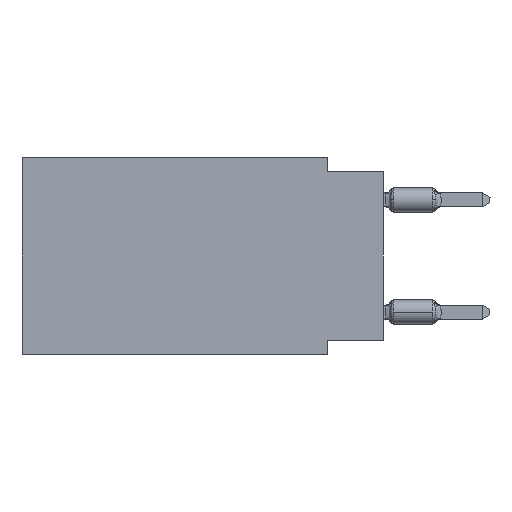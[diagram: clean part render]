
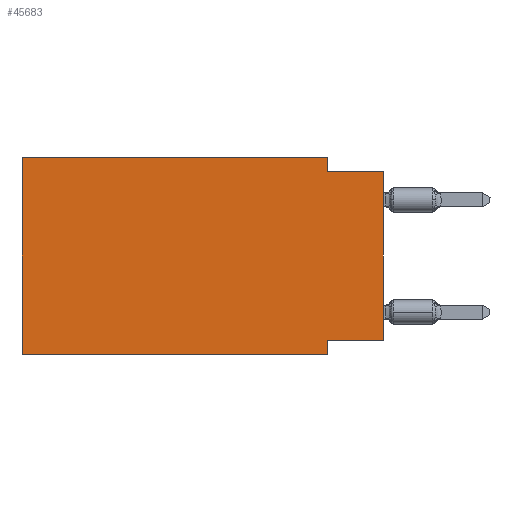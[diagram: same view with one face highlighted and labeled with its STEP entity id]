
A CAD part, left-side view. The second image highlights one B-rep face of the part: STEP entity #45683.
In plain terms, the highlighted planar face has unit normal (-1, 0, 0).
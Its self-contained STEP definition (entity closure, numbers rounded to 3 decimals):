
#59 = DIRECTION ( 'NONE',  ( 0., 0., -1. ) ) ;
#446 = FACE_OUTER_BOUND ( 'NONE', #4276, .T. ) ;
#1036 = LINE ( 'NONE', #35145, #41183 ) ;
#1537 = VECTOR ( 'NONE', #14599, 1000. ) ;
#4276 = EDGE_LOOP ( 'NONE', ( #37272, #40240, #27308, #10189, #48614, #50763, #18307, #34045 ) ) ;
#5012 = LINE ( 'NONE', #43557, #22860 ) ;
#5302 = DIRECTION ( 'NONE',  ( 0., 0., -1. ) ) ;
#6295 = LINE ( 'NONE', #26535, #19791 ) ;
#8601 = LINE ( 'NONE', #16154, #52052 ) ;
#10189 = ORIENTED_EDGE ( 'NONE', *, *, #12816, .F. ) ;
#10471 = LINE ( 'NONE', #44830, #11822 ) ;
#11822 = VECTOR ( 'NONE', #31735, 1000. ) ;
#11825 = CARTESIAN_POINT ( 'NONE',  ( 0., 2.54, -8.255 ) ) ;
#12816 = EDGE_CURVE ( 'NONE', #19224, #33314, #44764, .T. ) ;
#14599 = DIRECTION ( 'NONE',  ( 0., -1., 0. ) ) ;
#15136 = LINE ( 'NONE', #53991, #41627 ) ;
#16012 = VERTEX_POINT ( 'NONE', #49043 ) ;
#16154 = CARTESIAN_POINT ( 'NONE',  ( 0., 0., 0. ) ) ;
#16433 = DIRECTION ( 'NONE',  ( 0., 0., 1. ) ) ;
#16468 = CARTESIAN_POINT ( 'NONE',  ( 0., 16.383, 0. ) ) ;
#16653 = CARTESIAN_POINT ( 'NONE',  ( 0., 16.383, 0. ) ) ;
#17655 = LINE ( 'NONE', #38614, #36077 ) ;
#18260 = CARTESIAN_POINT ( 'NONE',  ( 0., 16.383, 0. ) ) ;
#18307 = ORIENTED_EDGE ( 'NONE', *, *, #51370, .F. ) ;
#18781 = VERTEX_POINT ( 'NONE', #11825 ) ;
#19181 = CARTESIAN_POINT ( 'NONE',  ( 0., 2.54, -0.635 ) ) ;
#19224 = VERTEX_POINT ( 'NONE', #16468 ) ;
#19791 = VECTOR ( 'NONE', #5302, 1000. ) ;
#21035 = EDGE_CURVE ( 'NONE', #38456, #48633, #10471, .T. ) ;
#21861 = EDGE_CURVE ( 'NONE', #33314, #38456, #17655, .T. ) ;
#22860 = VECTOR ( 'NONE', #35968, 1000. ) ;
#24431 = EDGE_CURVE ( 'NONE', #53372, #19224, #5012, .T. ) ;
#25414 = EDGE_CURVE ( 'NONE', #41303, #18781, #15136, .T. ) ;
#26211 = CARTESIAN_POINT ( 'NONE',  ( 0., 0., -0.635 ) ) ;
#26535 = CARTESIAN_POINT ( 'NONE',  ( 0., 2.54, -8.89 ) ) ;
#27308 = ORIENTED_EDGE ( 'NONE', *, *, #21861, .F. ) ;
#31735 = DIRECTION ( 'NONE',  ( 0., -1., 0. ) ) ;
#33314 = VERTEX_POINT ( 'NONE', #37011 ) ;
#34045 = ORIENTED_EDGE ( 'NONE', *, *, #25414, .F. ) ;
#35145 = CARTESIAN_POINT ( 'NONE',  ( 0., 16.383, -8.89 ) ) ;
#35968 = DIRECTION ( 'NONE',  ( 0., 0., 1. ) ) ;
#36077 = VECTOR ( 'NONE', #59, 1000. ) ;
#36387 = DIRECTION ( 'NONE',  ( 0., 1., 0. ) ) ;
#37011 = CARTESIAN_POINT ( 'NONE',  ( 0., 2.54, 0. ) ) ;
#37272 = ORIENTED_EDGE ( 'NONE', *, *, #52765, .T. ) ;
#37618 = DIRECTION ( 'NONE',  ( 1., 0., 0. ) ) ;
#38171 = PLANE ( 'NONE',  #53448 ) ;
#38456 = VERTEX_POINT ( 'NONE', #19181 ) ;
#38614 = CARTESIAN_POINT ( 'NONE',  ( 0., 2.54, 0. ) ) ;
#40240 = ORIENTED_EDGE ( 'NONE', *, *, #21035, .F. ) ;
#40260 = CARTESIAN_POINT ( 'NONE',  ( 0., 16.383, -8.89 ) ) ;
#41183 = VECTOR ( 'NONE', #52180, 1000. ) ;
#41303 = VERTEX_POINT ( 'NONE', #45433 ) ;
#41627 = VECTOR ( 'NONE', #36387, 1000. ) ;
#43557 = CARTESIAN_POINT ( 'NONE',  ( 0., 16.383, 0. ) ) ;
#44764 = LINE ( 'NONE', #18260, #1537 ) ;
#44830 = CARTESIAN_POINT ( 'NONE',  ( 0., 0., -0.635 ) ) ;
#45433 = CARTESIAN_POINT ( 'NONE',  ( 0., 0., -8.255 ) ) ;
#45683 = ADVANCED_FACE ( 'NONE', ( #446 ), #38171, .F. ) ;
#48614 = ORIENTED_EDGE ( 'NONE', *, *, #24431, .F. ) ;
#48633 = VERTEX_POINT ( 'NONE', #26211 ) ;
#49043 = CARTESIAN_POINT ( 'NONE',  ( 0., 2.54, -8.89 ) ) ;
#50763 = ORIENTED_EDGE ( 'NONE', *, *, #51037, .T. ) ;
#51026 = DIRECTION ( 'NONE',  ( 0., 0., -1. ) ) ;
#51037 = EDGE_CURVE ( 'NONE', #53372, #16012, #1036, .T. ) ;
#51370 = EDGE_CURVE ( 'NONE', #18781, #16012, #6295, .T. ) ;
#52052 = VECTOR ( 'NONE', #16433, 1000. ) ;
#52180 = DIRECTION ( 'NONE',  ( 0., -1., 0. ) ) ;
#52765 = EDGE_CURVE ( 'NONE', #41303, #48633, #8601, .T. ) ;
#53372 = VERTEX_POINT ( 'NONE', #40260 ) ;
#53448 = AXIS2_PLACEMENT_3D ( 'NONE', #16653, #37618, #51026 ) ;
#53991 = CARTESIAN_POINT ( 'NONE',  ( 0., 0., -8.255 ) ) ;
